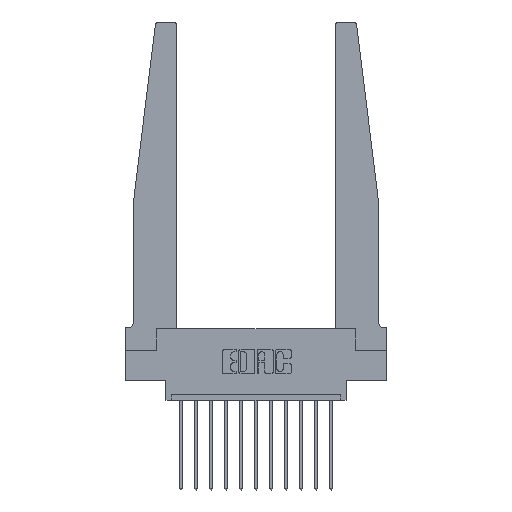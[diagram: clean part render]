
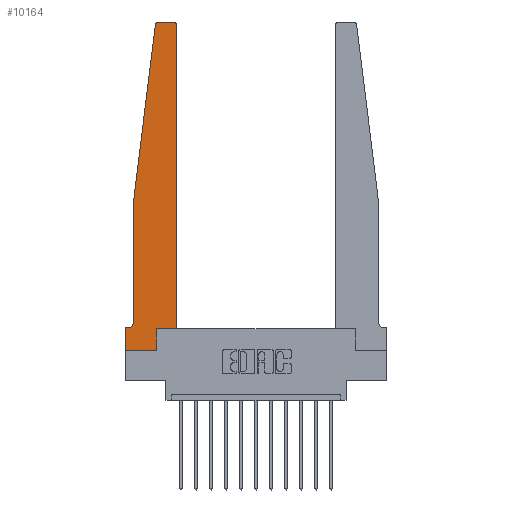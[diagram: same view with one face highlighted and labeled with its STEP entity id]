
A CAD part, top view. The second image highlights one B-rep face of the part: STEP entity #10164.
In plain terms, the highlighted planar face has unit normal (0, 0, 1).
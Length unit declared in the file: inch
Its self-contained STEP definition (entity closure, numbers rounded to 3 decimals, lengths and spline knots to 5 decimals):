
#344 = DIRECTION ( 'NONE',  ( 1., 0., 0. ) ) ;
#719 = VERTEX_POINT ( 'NONE', #5376 ) ;
#810 = CARTESIAN_POINT ( 'NONE',  ( 0.065, 1.25, 0.37 ) ) ;
#1031 = VECTOR ( 'NONE', #6439, 39.37008 ) ;
#1089 = VERTEX_POINT ( 'NONE', #6477 ) ;
#1181 = PLANE ( 'NONE',  #5861 ) ;
#1247 = DIRECTION ( 'NONE',  ( 0., -1., 0. ) ) ;
#1262 = VERTEX_POINT ( 'NONE', #11575 ) ;
#1303 = VECTOR ( 'NONE', #8026, 39.37008 ) ;
#1490 = VERTEX_POINT ( 'NONE', #14991 ) ;
#1581 = LINE ( 'NONE', #15207, #16123 ) ;
#1611 = DIRECTION ( 'NONE',  ( 1., 0., 0. ) ) ;
#1647 = DIRECTION ( 'NONE',  ( 1., 0., 0. ) ) ;
#1858 = LINE ( 'NONE', #14576, #15645 ) ;
#1948 = DIRECTION ( 'NONE',  ( 0., 0., -1. ) ) ;
#1972 = CARTESIAN_POINT ( 'NONE',  ( 0.065, 0.1875, 0.37 ) ) ;
#2061 = VECTOR ( 'NONE', #344, 39.37008 ) ;
#2068 = EDGE_CURVE ( 'NONE', #3778, #1490, #5927, .T. ) ;
#2127 = CIRCLE ( 'NONE', #7136, 0.03 ) ;
#2326 = AXIS2_PLACEMENT_3D ( 'NONE', #3962, #7740, #1647 ) ;
#2645 = AXIS2_PLACEMENT_3D ( 'NONE', #15811, #1948, #12169 ) ;
#2674 = DIRECTION ( 'NONE',  ( 1., 0., 0. ) ) ;
#2692 = DIRECTION ( 'NONE',  ( 0., 0., 1. ) ) ;
#2716 = ORIENTED_EDGE ( 'NONE', *, *, #12839, .T. ) ;
#3006 = LINE ( 'NONE', #12912, #1303 ) ;
#3064 = CARTESIAN_POINT ( 'NONE',  ( 0., 0., 0.37 ) ) ;
#3179 = ORIENTED_EDGE ( 'NONE', *, *, #2068, .T. ) ;
#3459 = CARTESIAN_POINT ( 'NONE',  ( 0.425, 0.18, 0.37 ) ) ;
#3778 = VERTEX_POINT ( 'NONE', #6554 ) ;
#3962 = CARTESIAN_POINT ( 'NONE',  ( 0.27653, 2.72, 0.37 ) ) ;
#4756 = DIRECTION ( 'NONE',  ( -0.122, -0.992, 0. ) ) ;
#4849 = ORIENTED_EDGE ( 'NONE', *, *, #11927, .T. ) ;
#5101 = LINE ( 'NONE', #10134, #14078 ) ;
#5130 = ORIENTED_EDGE ( 'NONE', *, *, #14162, .T. ) ;
#5376 = CARTESIAN_POINT ( 'NONE',  ( 0.065, 0.2375, 0.37 ) ) ;
#5547 = EDGE_CURVE ( 'NONE', #1089, #9433, #9327, .T. ) ;
#5566 = DIRECTION ( 'NONE',  ( 0., 1., 0. ) ) ;
#5861 = AXIS2_PLACEMENT_3D ( 'NONE', #12492, #11413, #2674 ) ;
#5927 = LINE ( 'NONE', #9914, #7458 ) ;
#6051 = CIRCLE ( 'NONE', #2326, 0.03 ) ;
#6251 = CARTESIAN_POINT ( 'NONE',  ( 0.015, 0.1875, 0.37 ) ) ;
#6401 = FACE_OUTER_BOUND ( 'NONE', #10865, .T. ) ;
#6439 = DIRECTION ( 'NONE',  ( 0., 1., 0. ) ) ;
#6472 = VERTEX_POINT ( 'NONE', #10112 ) ;
#6477 = CARTESIAN_POINT ( 'NONE',  ( 0., 0., 0.37 ) ) ;
#6554 = CARTESIAN_POINT ( 'NONE',  ( 0.395, 2.75, 0.37 ) ) ;
#6699 = ORIENTED_EDGE ( 'NONE', *, *, #8312, .T. ) ;
#6851 = CARTESIAN_POINT ( 'NONE',  ( 0.065, 1.25, 0.37 ) ) ;
#7136 = AXIS2_PLACEMENT_3D ( 'NONE', #13994, #2692, #1611 ) ;
#7458 = VECTOR ( 'NONE', #8604, 39.37008 ) ;
#7606 = VERTEX_POINT ( 'NONE', #10373 ) ;
#7740 = DIRECTION ( 'NONE',  ( 0., 0., 1. ) ) ;
#7883 = EDGE_CURVE ( 'NONE', #719, #8629, #10535, .T. ) ;
#8026 = DIRECTION ( 'NONE',  ( 0., -1., 0. ) ) ;
#8158 = VERTEX_POINT ( 'NONE', #6851 ) ;
#8312 = EDGE_CURVE ( 'NONE', #12768, #9395, #8883, .T. ) ;
#8465 = ORIENTED_EDGE ( 'NONE', *, *, #12387, .T. ) ;
#8604 = DIRECTION ( 'NONE',  ( -1., 0., 0. ) ) ;
#8629 = VERTEX_POINT ( 'NONE', #6251 ) ;
#8770 = EDGE_CURVE ( 'NONE', #9395, #3778, #2127, .T. ) ;
#8883 = LINE ( 'NONE', #15094, #1031 ) ;
#9327 = LINE ( 'NONE', #3064, #2061 ) ;
#9378 = ORIENTED_EDGE ( 'NONE', *, *, #7883, .T. ) ;
#9395 = VERTEX_POINT ( 'NONE', #11279 ) ;
#9433 = VERTEX_POINT ( 'NONE', #13187 ) ;
#9914 = CARTESIAN_POINT ( 'NONE',  ( 0.25, 2.75, 0.37 ) ) ;
#10112 = CARTESIAN_POINT ( 'NONE',  ( 0., 0.1875, 0.37 ) ) ;
#10134 = CARTESIAN_POINT ( 'NONE',  ( 0.425, 0.18, 0.37 ) ) ;
#10164 = ADVANCED_FACE ( 'NONE', ( #6401 ), #1181, .T. ) ;
#10373 = CARTESIAN_POINT ( 'NONE',  ( 0.24675, 2.72367, 0.37 ) ) ;
#10535 = CIRCLE ( 'NONE', #2645, 0.05 ) ;
#10865 = EDGE_LOOP ( 'NONE', ( #3179, #5130, #15204, #14926, #9378, #4849, #14350, #15686, #8465, #2716, #6699, #12087 ) ) ;
#11032 = LINE ( 'NONE', #810, #14851 ) ;
#11279 = CARTESIAN_POINT ( 'NONE',  ( 0.425, 2.72, 0.37 ) ) ;
#11413 = DIRECTION ( 'NONE',  ( 0., 0., 1. ) ) ;
#11575 = CARTESIAN_POINT ( 'NONE',  ( 0.2605, 0.18, 0.37 ) ) ;
#11787 = DIRECTION ( 'NONE',  ( -1., 0., 0. ) ) ;
#11927 = EDGE_CURVE ( 'NONE', #8629, #6472, #15752, .T. ) ;
#12087 = ORIENTED_EDGE ( 'NONE', *, *, #8770, .T. ) ;
#12169 = DIRECTION ( 'NONE',  ( -1., 0., 0. ) ) ;
#12387 = EDGE_CURVE ( 'NONE', #9433, #1262, #1858, .T. ) ;
#12492 = CARTESIAN_POINT ( 'NONE',  ( 0., 0.1875, 0.37 ) ) ;
#12768 = VERTEX_POINT ( 'NONE', #3459 ) ;
#12839 = EDGE_CURVE ( 'NONE', #1262, #12768, #5101, .T. ) ;
#12912 = CARTESIAN_POINT ( 'NONE',  ( 0., 0., 0.37 ) ) ;
#13187 = CARTESIAN_POINT ( 'NONE',  ( 0.2605, 0., 0.37 ) ) ;
#13242 = EDGE_CURVE ( 'NONE', #7606, #8158, #11032, .T. ) ;
#13875 = EDGE_CURVE ( 'NONE', #6472, #1089, #3006, .T. ) ;
#13994 = CARTESIAN_POINT ( 'NONE',  ( 0.395, 2.72, 0.37 ) ) ;
#14078 = VECTOR ( 'NONE', #15194, 39.37008 ) ;
#14162 = EDGE_CURVE ( 'NONE', #1490, #7606, #6051, .T. ) ;
#14325 = VECTOR ( 'NONE', #11787, 39.37008 ) ;
#14350 = ORIENTED_EDGE ( 'NONE', *, *, #13875, .T. ) ;
#14576 = CARTESIAN_POINT ( 'NONE',  ( 0.2605, 0.18, 0.37 ) ) ;
#14851 = VECTOR ( 'NONE', #4756, 39.37008 ) ;
#14926 = ORIENTED_EDGE ( 'NONE', *, *, #16150, .T. ) ;
#14991 = CARTESIAN_POINT ( 'NONE',  ( 0.27653, 2.75, 0.37 ) ) ;
#15094 = CARTESIAN_POINT ( 'NONE',  ( 0.425, 0.18, 0.37 ) ) ;
#15194 = DIRECTION ( 'NONE',  ( 1., 0., 0. ) ) ;
#15204 = ORIENTED_EDGE ( 'NONE', *, *, #13242, .T. ) ;
#15207 = CARTESIAN_POINT ( 'NONE',  ( 0.065, 1.25, 0.37 ) ) ;
#15645 = VECTOR ( 'NONE', #5566, 39.37008 ) ;
#15686 = ORIENTED_EDGE ( 'NONE', *, *, #5547, .T. ) ;
#15752 = LINE ( 'NONE', #1972, #14325 ) ;
#15811 = CARTESIAN_POINT ( 'NONE',  ( 0.015, 0.2375, 0.37 ) ) ;
#16123 = VECTOR ( 'NONE', #1247, 39.37008 ) ;
#16150 = EDGE_CURVE ( 'NONE', #8158, #719, #1581, .T. ) ;
